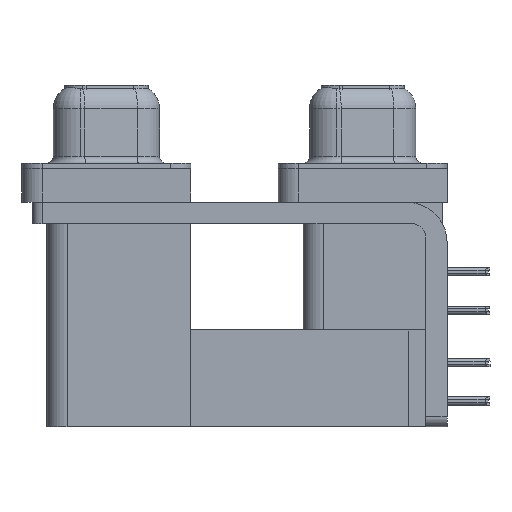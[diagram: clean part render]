
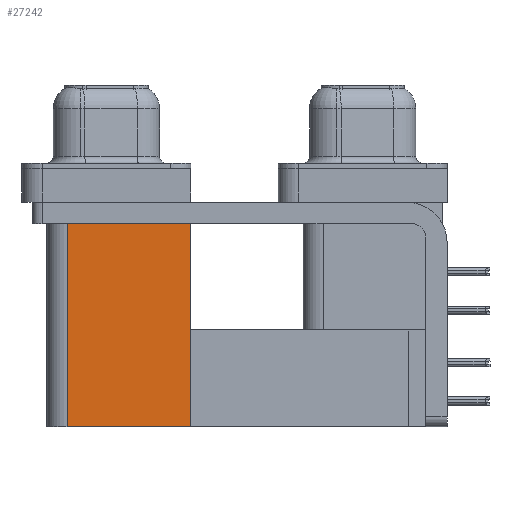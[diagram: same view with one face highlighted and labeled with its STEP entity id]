
A CAD part, left-side view. The second image highlights one B-rep face of the part: STEP entity #27242.
In plain terms, the highlighted planar face has unit normal (-1, 0, 0).
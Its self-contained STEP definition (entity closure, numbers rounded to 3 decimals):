
#1255 = CARTESIAN_POINT ( 'NONE',  ( 3.765, 12.775, -19.2 ) ) ;
#2138 = EDGE_CURVE ( 'NONE', #47312, #20278, #30127, .T. ) ;
#5601 = DIRECTION ( 'NONE',  ( 0., 0., 1. ) ) ;
#6342 = CARTESIAN_POINT ( 'NONE',  ( 3.765, 21.975, -19.2 ) ) ;
#6812 = DIRECTION ( 'NONE',  ( 1., 0., 0. ) ) ;
#11697 = LINE ( 'NONE', #15642, #30916 ) ;
#12864 = VECTOR ( 'NONE', #42213, 1000. ) ;
#13506 = PLANE ( 'NONE',  #20888 ) ;
#14482 = CARTESIAN_POINT ( 'NONE',  ( 3.765, 21.975, -19.2 ) ) ;
#15642 = CARTESIAN_POINT ( 'NONE',  ( 3.765, 12.775, -19.2 ) ) ;
#16713 = FACE_OUTER_BOUND ( 'NONE', #34311, .T. ) ;
#17444 = ORIENTED_EDGE ( 'NONE', *, *, #20925, .F. ) ;
#17484 = VERTEX_POINT ( 'NONE', #25111 ) ;
#17853 = EDGE_CURVE ( 'NONE', #17484, #47312, #11697, .T. ) ;
#19554 = CARTESIAN_POINT ( 'NONE',  ( 3.765, 21.975, -2.5 ) ) ;
#20278 = VERTEX_POINT ( 'NONE', #19554 ) ;
#20888 = AXIS2_PLACEMENT_3D ( 'NONE', #40372, #6812, #47027 ) ;
#20925 = EDGE_CURVE ( 'NONE', #17484, #35919, #34595, .T. ) ;
#25111 = CARTESIAN_POINT ( 'NONE',  ( 3.765, 12.775, -19.2 ) ) ;
#27156 = CARTESIAN_POINT ( 'NONE',  ( 3.765, 12.775, -2.5 ) ) ;
#27242 = ADVANCED_FACE ( 'NONE', ( #16713 ), #13506, .F. ) ;
#29734 = CARTESIAN_POINT ( 'NONE',  ( 3.765, 12.775, -2.5 ) ) ;
#30127 = LINE ( 'NONE', #27156, #32327 ) ;
#30916 = VECTOR ( 'NONE', #34144, 1000. ) ;
#31487 = ORIENTED_EDGE ( 'NONE', *, *, #38609, .F. ) ;
#32327 = VECTOR ( 'NONE', #45155, 1000. ) ;
#34144 = DIRECTION ( 'NONE',  ( 0., 0., 1. ) ) ;
#34311 = EDGE_LOOP ( 'NONE', ( #36794, #31487, #17444, #46682 ) ) ;
#34595 = LINE ( 'NONE', #1255, #12864 ) ;
#35264 = VECTOR ( 'NONE', #5601, 1000. ) ;
#35919 = VERTEX_POINT ( 'NONE', #14482 ) ;
#36794 = ORIENTED_EDGE ( 'NONE', *, *, #2138, .T. ) ;
#38609 = EDGE_CURVE ( 'NONE', #35919, #20278, #39890, .T. ) ;
#39890 = LINE ( 'NONE', #6342, #35264 ) ;
#40372 = CARTESIAN_POINT ( 'NONE',  ( 3.765, 12.775, -19.2 ) ) ;
#42213 = DIRECTION ( 'NONE',  ( 0., 1., 0. ) ) ;
#45155 = DIRECTION ( 'NONE',  ( 0., 1., 0. ) ) ;
#46682 = ORIENTED_EDGE ( 'NONE', *, *, #17853, .T. ) ;
#47027 = DIRECTION ( 'NONE',  ( 0., 0., -1. ) ) ;
#47312 = VERTEX_POINT ( 'NONE', #29734 ) ;
